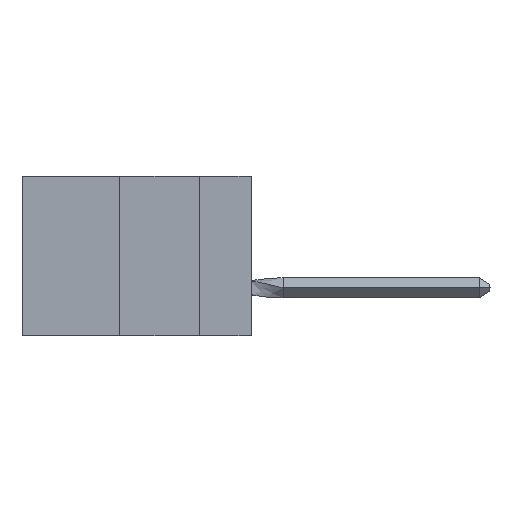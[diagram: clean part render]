
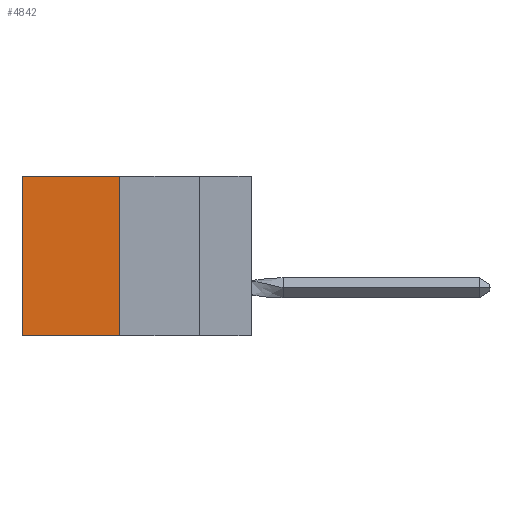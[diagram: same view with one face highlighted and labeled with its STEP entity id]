
A CAD part, left-side view. The second image highlights one B-rep face of the part: STEP entity #4842.
In plain terms, the highlighted planar face has unit normal (-1, 0, 0).
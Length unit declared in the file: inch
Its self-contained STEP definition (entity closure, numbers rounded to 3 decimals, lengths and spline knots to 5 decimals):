
#195 = EDGE_LOOP ( 'NONE', ( #7707, #8083, #5072, #12413 ) ) ;
#299 = DIRECTION ( 'NONE',  ( 0., 0., -1. ) ) ;
#498 = CARTESIAN_POINT ( 'NONE',  ( 0.305, 0.413, 0. ) ) ;
#624 = LINE ( 'NONE', #1323, #8811 ) ;
#825 = CARTESIAN_POINT ( 'NONE',  ( 0.305, 0.413, -0.5 ) ) ;
#1323 = CARTESIAN_POINT ( 'NONE',  ( 0.305, 0.413, -0.5 ) ) ;
#1457 = EDGE_CURVE ( 'NONE', #13261, #9671, #13683, .T. ) ;
#1611 = DIRECTION ( 'NONE',  ( 0., 1., 0. ) ) ;
#3390 = VECTOR ( 'NONE', #13540, 39.37008 ) ;
#3507 = CARTESIAN_POINT ( 'NONE',  ( 0.305, 0.72, -0.5 ) ) ;
#3636 = AXIS2_PLACEMENT_3D ( 'NONE', #9270, #5800, #13304 ) ;
#3674 = CARTESIAN_POINT ( 'NONE',  ( 0.305, 0.413, -0.5 ) ) ;
#4127 = VECTOR ( 'NONE', #9747, 39.37008 ) ;
#4460 = CARTESIAN_POINT ( 'NONE',  ( 0.305, 0.72, -0.5 ) ) ;
#4485 = FACE_OUTER_BOUND ( 'NONE', #195, .T. ) ;
#4842 = ADVANCED_FACE ( 'NONE', ( #4485 ), #9159, .F. ) ;
#5072 = ORIENTED_EDGE ( 'NONE', *, *, #6279, .F. ) ;
#5124 = VERTEX_POINT ( 'NONE', #7350 ) ;
#5566 = EDGE_CURVE ( 'NONE', #7090, #5124, #8279, .T. ) ;
#5800 = DIRECTION ( 'NONE',  ( 1., 0., 0. ) ) ;
#6279 = EDGE_CURVE ( 'NONE', #7090, #13261, #624, .T. ) ;
#7090 = VERTEX_POINT ( 'NONE', #498 ) ;
#7350 = CARTESIAN_POINT ( 'NONE',  ( 0.305, 0.72, 0. ) ) ;
#7707 = ORIENTED_EDGE ( 'NONE', *, *, #9665, .T. ) ;
#8083 = ORIENTED_EDGE ( 'NONE', *, *, #1457, .F. ) ;
#8279 = LINE ( 'NONE', #12394, #13733 ) ;
#8811 = VECTOR ( 'NONE', #299, 39.37008 ) ;
#9159 = PLANE ( 'NONE',  #3636 ) ;
#9270 = CARTESIAN_POINT ( 'NONE',  ( 0.305, 0.413, -0.5 ) ) ;
#9665 = EDGE_CURVE ( 'NONE', #5124, #9671, #9793, .T. ) ;
#9671 = VERTEX_POINT ( 'NONE', #3507 ) ;
#9747 = DIRECTION ( 'NONE',  ( 0., 0., -1. ) ) ;
#9793 = LINE ( 'NONE', #4460, #4127 ) ;
#12394 = CARTESIAN_POINT ( 'NONE',  ( 0.305, 0.413, 0. ) ) ;
#12413 = ORIENTED_EDGE ( 'NONE', *, *, #5566, .T. ) ;
#13261 = VERTEX_POINT ( 'NONE', #3674 ) ;
#13304 = DIRECTION ( 'NONE',  ( 0., 0., -1. ) ) ;
#13540 = DIRECTION ( 'NONE',  ( 0., 1., 0. ) ) ;
#13683 = LINE ( 'NONE', #825, #3390 ) ;
#13733 = VECTOR ( 'NONE', #1611, 39.37008 ) ;
